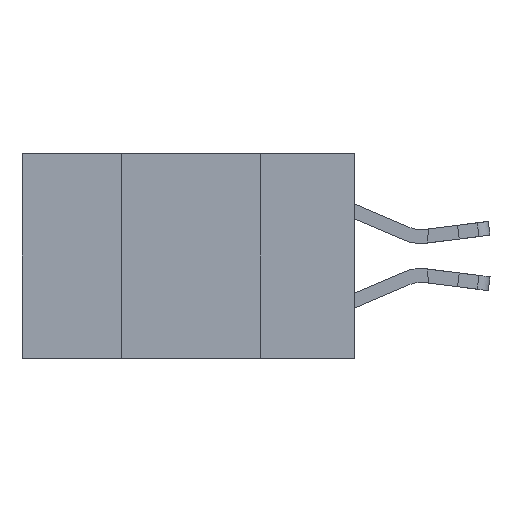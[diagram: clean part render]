
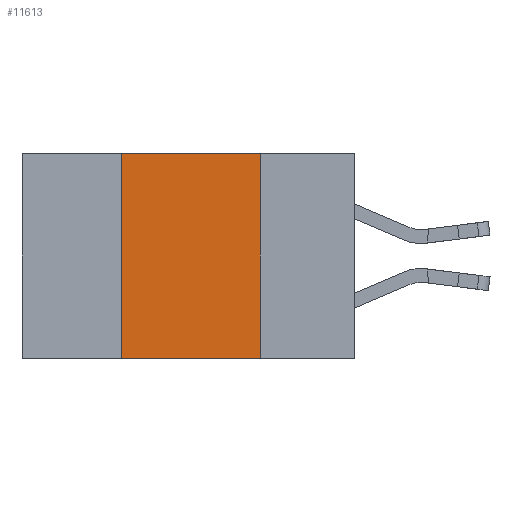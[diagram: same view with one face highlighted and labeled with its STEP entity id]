
A CAD part, left-side view. The second image highlights one B-rep face of the part: STEP entity #11613.
In plain terms, the highlighted planar face has unit normal (-1, 0, 0).
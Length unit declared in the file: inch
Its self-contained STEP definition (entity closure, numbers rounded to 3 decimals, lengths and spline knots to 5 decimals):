
#803 = ORIENTED_EDGE ( 'NONE', *, *, #13026, .T. ) ;
#1394 = VERTEX_POINT ( 'NONE', #16942 ) ;
#2130 = DIRECTION ( 'NONE',  ( 0., -1., 0. ) ) ;
#2312 = LINE ( 'NONE', #3499, #21938 ) ;
#2392 = FACE_OUTER_BOUND ( 'NONE', #2685, .T. ) ;
#2661 = LINE ( 'NONE', #27089, #13558 ) ;
#2685 = EDGE_LOOP ( 'NONE', ( #28494, #17223, #23004, #803 ) ) ;
#3499 = CARTESIAN_POINT ( 'NONE',  ( 0., 0.17, 0. ) ) ;
#5784 = DIRECTION ( 'NONE',  ( 0., 0., -1. ) ) ;
#9239 = AXIS2_PLACEMENT_3D ( 'NONE', #19451, #14568, #10731 ) ;
#10731 = DIRECTION ( 'NONE',  ( 0., 0., -1. ) ) ;
#10985 = CARTESIAN_POINT ( 'NONE',  ( 0., 0.17, 0. ) ) ;
#11613 = ADVANCED_FACE ( 'NONE', ( #2392 ), #17032, .F. ) ;
#11650 = DIRECTION ( 'NONE',  ( 0., 0., 1. ) ) ;
#13026 = EDGE_CURVE ( 'NONE', #1394, #16344, #2661, .T. ) ;
#13558 = VECTOR ( 'NONE', #2130, 39.37008 ) ;
#14568 = DIRECTION ( 'NONE',  ( 1., 0., 0. ) ) ;
#14908 = EDGE_CURVE ( 'NONE', #1394, #16920, #19361, .T. ) ;
#15129 = CARTESIAN_POINT ( 'NONE',  ( 0., 0.42, 0. ) ) ;
#16344 = VERTEX_POINT ( 'NONE', #27867 ) ;
#16663 = LINE ( 'NONE', #27033, #18748 ) ;
#16920 = VERTEX_POINT ( 'NONE', #15129 ) ;
#16942 = CARTESIAN_POINT ( 'NONE',  ( 0., 0.42, -0.37 ) ) ;
#17032 = PLANE ( 'NONE',  #9239 ) ;
#17223 = ORIENTED_EDGE ( 'NONE', *, *, #21959, .F. ) ;
#18748 = VECTOR ( 'NONE', #26936, 39.37008 ) ;
#19361 = LINE ( 'NONE', #25012, #23569 ) ;
#19451 = CARTESIAN_POINT ( 'NONE',  ( 0., 0.6, 0. ) ) ;
#21938 = VECTOR ( 'NONE', #5784, 39.37008 ) ;
#21959 = EDGE_CURVE ( 'NONE', #16920, #26022, #16663, .T. ) ;
#23004 = ORIENTED_EDGE ( 'NONE', *, *, #14908, .F. ) ;
#23569 = VECTOR ( 'NONE', #11650, 39.37008 ) ;
#25012 = CARTESIAN_POINT ( 'NONE',  ( 0., 0.42, 0. ) ) ;
#26022 = VERTEX_POINT ( 'NONE', #10985 ) ;
#26936 = DIRECTION ( 'NONE',  ( 0., -1., 0. ) ) ;
#27033 = CARTESIAN_POINT ( 'NONE',  ( 0., 0.6, 0. ) ) ;
#27089 = CARTESIAN_POINT ( 'NONE',  ( 0., 0.6, -0.37 ) ) ;
#27154 = EDGE_CURVE ( 'NONE', #26022, #16344, #2312, .T. ) ;
#27867 = CARTESIAN_POINT ( 'NONE',  ( 0., 0.17, -0.37 ) ) ;
#28494 = ORIENTED_EDGE ( 'NONE', *, *, #27154, .F. ) ;
